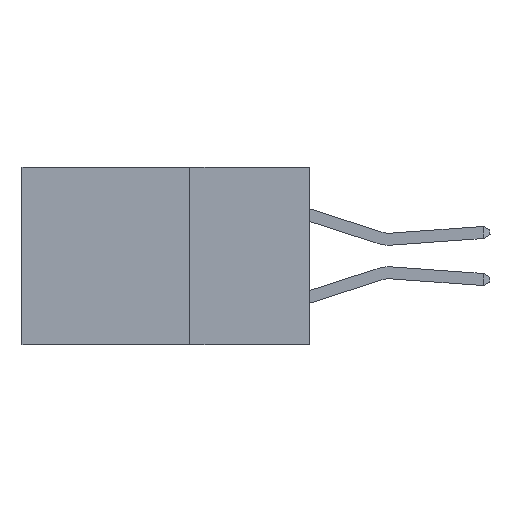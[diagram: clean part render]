
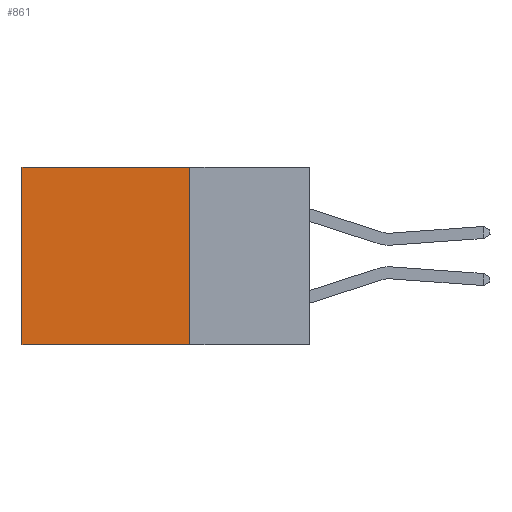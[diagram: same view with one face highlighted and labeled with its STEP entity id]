
A CAD part, left-side view. The second image highlights one B-rep face of the part: STEP entity #861.
In plain terms, the highlighted planar face has unit normal (-1, 0, 0).
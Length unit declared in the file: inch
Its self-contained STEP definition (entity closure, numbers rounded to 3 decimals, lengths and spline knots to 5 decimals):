
#10 = CARTESIAN_POINT ( 'NONE',  ( 0.2615, 0.25, 0. ) ) ;
#117 = VERTEX_POINT ( 'NONE', #10877 ) ;
#410 = VECTOR ( 'NONE', #2902, 39.37008 ) ;
#499 = LINE ( 'NONE', #635, #1446 ) ;
#635 = CARTESIAN_POINT ( 'NONE',  ( 0.2615, 0.25, -0.37 ) ) ;
#861 = ADVANCED_FACE ( 'NONE', ( #1174 ), #8087, .F. ) ;
#1093 = ORIENTED_EDGE ( 'NONE', *, *, #9234, .T. ) ;
#1174 = FACE_OUTER_BOUND ( 'NONE', #5196, .T. ) ;
#1446 = VECTOR ( 'NONE', #4495, 39.37008 ) ;
#2452 = CARTESIAN_POINT ( 'NONE',  ( 0.2615, 0.25, -0.37 ) ) ;
#2902 = DIRECTION ( 'NONE',  ( 0., 1., 0. ) ) ;
#3147 = ORIENTED_EDGE ( 'NONE', *, *, #8637, .F. ) ;
#3382 = VERTEX_POINT ( 'NONE', #10702 ) ;
#3528 = AXIS2_PLACEMENT_3D ( 'NONE', #9131, #6134, #5159 ) ;
#3875 = LINE ( 'NONE', #11838, #410 ) ;
#4007 = CARTESIAN_POINT ( 'NONE',  ( 0.2615, 0.6, -0.37 ) ) ;
#4495 = DIRECTION ( 'NONE',  ( 0., 0., -1. ) ) ;
#4554 = LINE ( 'NONE', #2452, #5009 ) ;
#4851 = VERTEX_POINT ( 'NONE', #10 ) ;
#5009 = VECTOR ( 'NONE', #7678, 39.37008 ) ;
#5159 = DIRECTION ( 'NONE',  ( 0., 0., -1. ) ) ;
#5196 = EDGE_LOOP ( 'NONE', ( #1093, #12379, #3147, #10752 ) ) ;
#5967 = LINE ( 'NONE', #4007, #7509 ) ;
#6134 = DIRECTION ( 'NONE',  ( 1., 0., 0. ) ) ;
#7509 = VECTOR ( 'NONE', #9692, 39.37008 ) ;
#7678 = DIRECTION ( 'NONE',  ( 0., 1., 0. ) ) ;
#7821 = VERTEX_POINT ( 'NONE', #8884 ) ;
#8087 = PLANE ( 'NONE',  #3528 ) ;
#8637 = EDGE_CURVE ( 'NONE', #4851, #117, #499, .T. ) ;
#8645 = EDGE_CURVE ( 'NONE', #117, #3382, #4554, .T. ) ;
#8884 = CARTESIAN_POINT ( 'NONE',  ( 0.2615, 0.6, 0. ) ) ;
#9131 = CARTESIAN_POINT ( 'NONE',  ( 0.2615, 0.25, -0.37 ) ) ;
#9234 = EDGE_CURVE ( 'NONE', #7821, #3382, #5967, .T. ) ;
#9361 = EDGE_CURVE ( 'NONE', #4851, #7821, #3875, .T. ) ;
#9692 = DIRECTION ( 'NONE',  ( 0., 0., -1. ) ) ;
#10702 = CARTESIAN_POINT ( 'NONE',  ( 0.2615, 0.6, -0.37 ) ) ;
#10752 = ORIENTED_EDGE ( 'NONE', *, *, #9361, .T. ) ;
#10877 = CARTESIAN_POINT ( 'NONE',  ( 0.2615, 0.25, -0.37 ) ) ;
#11838 = CARTESIAN_POINT ( 'NONE',  ( 0.2615, 0.25, 0. ) ) ;
#12379 = ORIENTED_EDGE ( 'NONE', *, *, #8645, .F. ) ;
